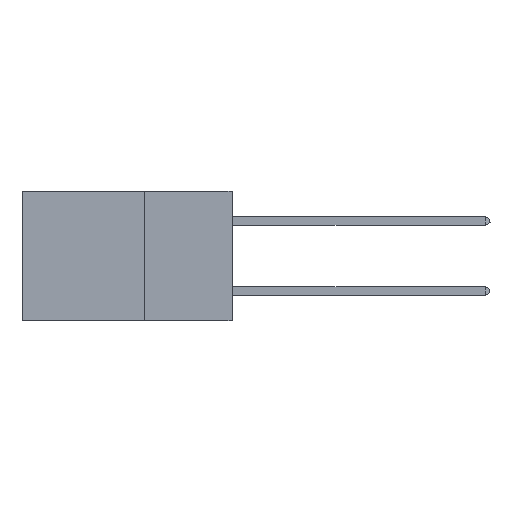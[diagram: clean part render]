
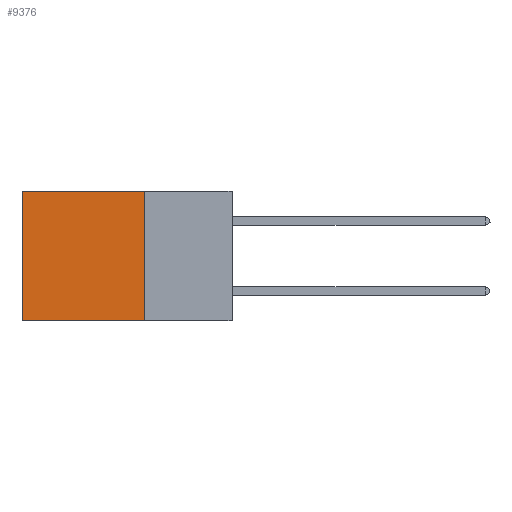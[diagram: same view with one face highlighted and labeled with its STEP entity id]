
A CAD part, left-side view. The second image highlights one B-rep face of the part: STEP entity #9376.
In plain terms, the highlighted planar face has unit normal (-1, 0, 0).
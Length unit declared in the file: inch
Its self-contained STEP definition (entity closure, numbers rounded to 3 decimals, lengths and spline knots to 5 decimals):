
#417 = CARTESIAN_POINT ( 'NONE',  ( 0.2875, 0.6, -0.37 ) ) ;
#665 = LINE ( 'NONE', #5888, #4142 ) ;
#1151 = CARTESIAN_POINT ( 'NONE',  ( 0.2875, 0.25, 0. ) ) ;
#1322 = CARTESIAN_POINT ( 'NONE',  ( 0.2875, 0.25, -0.37 ) ) ;
#1356 = VERTEX_POINT ( 'NONE', #1151 ) ;
#1549 = ORIENTED_EDGE ( 'NONE', *, *, #8776, .T. ) ;
#2658 = VECTOR ( 'NONE', #17634, 39.37008 ) ;
#2775 = CARTESIAN_POINT ( 'NONE',  ( 0.2875, 0.6, 0. ) ) ;
#2800 = VECTOR ( 'NONE', #8829, 39.37008 ) ;
#2966 = EDGE_CURVE ( 'NONE', #1356, #6134, #7495, .T. ) ;
#4142 = VECTOR ( 'NONE', #18119, 39.37008 ) ;
#5470 = DIRECTION ( 'NONE',  ( 1., 0., 0. ) ) ;
#5888 = CARTESIAN_POINT ( 'NONE',  ( 0.2875, 0.25, 0. ) ) ;
#6088 = DIRECTION ( 'NONE',  ( 0., 0., -1. ) ) ;
#6134 = VERTEX_POINT ( 'NONE', #1322 ) ;
#6979 = ORIENTED_EDGE ( 'NONE', *, *, #2966, .F. ) ;
#7160 = EDGE_LOOP ( 'NONE', ( #13675, #8660, #6979, #1549 ) ) ;
#7495 = LINE ( 'NONE', #13045, #2658 ) ;
#8345 = LINE ( 'NONE', #2775, #19973 ) ;
#8660 = ORIENTED_EDGE ( 'NONE', *, *, #14445, .F. ) ;
#8776 = EDGE_CURVE ( 'NONE', #1356, #8979, #665, .T. ) ;
#8829 = DIRECTION ( 'NONE',  ( 0., 1., 0. ) ) ;
#8979 = VERTEX_POINT ( 'NONE', #11207 ) ;
#9376 = ADVANCED_FACE ( 'NONE', ( #17122 ), #17652, .F. ) ;
#10065 = VERTEX_POINT ( 'NONE', #417 ) ;
#11207 = CARTESIAN_POINT ( 'NONE',  ( 0.2875, 0.6, 0. ) ) ;
#11682 = LINE ( 'NONE', #14867, #2800 ) ;
#13045 = CARTESIAN_POINT ( 'NONE',  ( 0.2875, 0.25, 0. ) ) ;
#13675 = ORIENTED_EDGE ( 'NONE', *, *, #14639, .T. ) ;
#14445 = EDGE_CURVE ( 'NONE', #6134, #10065, #11682, .T. ) ;
#14639 = EDGE_CURVE ( 'NONE', #8979, #10065, #8345, .T. ) ;
#14654 = CARTESIAN_POINT ( 'NONE',  ( 0.2875, 0.25, 0. ) ) ;
#14867 = CARTESIAN_POINT ( 'NONE',  ( 0.2875, 0.25, -0.37 ) ) ;
#16193 = DIRECTION ( 'NONE',  ( 0., 0., -1. ) ) ;
#16425 = AXIS2_PLACEMENT_3D ( 'NONE', #14654, #5470, #16193 ) ;
#17122 = FACE_OUTER_BOUND ( 'NONE', #7160, .T. ) ;
#17634 = DIRECTION ( 'NONE',  ( 0., 0., -1. ) ) ;
#17652 = PLANE ( 'NONE',  #16425 ) ;
#18119 = DIRECTION ( 'NONE',  ( 0., 1., 0. ) ) ;
#19973 = VECTOR ( 'NONE', #6088, 39.37008 ) ;
